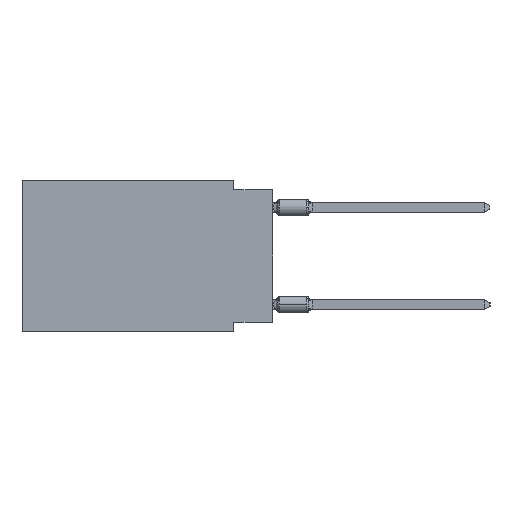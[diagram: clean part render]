
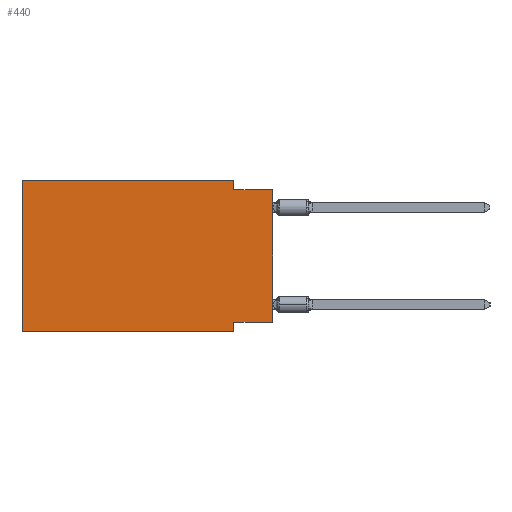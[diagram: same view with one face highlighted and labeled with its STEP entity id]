
A CAD part, left-side view. The second image highlights one B-rep face of the part: STEP entity #440.
In plain terms, the highlighted planar face has unit normal (-1, 0, 0).
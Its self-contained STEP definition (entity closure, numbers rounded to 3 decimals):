
#440 = ADVANCED_FACE ( 'NONE', ( #2501 ), #32997, .F. ) ;
#1200 = LINE ( 'NONE', #47412, #42851 ) ;
#1659 = DIRECTION ( 'NONE',  ( 0., 0., 1. ) ) ;
#2501 = FACE_OUTER_BOUND ( 'NONE', #46681, .T. ) ;
#2604 = CARTESIAN_POINT ( 'NONE',  ( 0., 16.383, 0. ) ) ;
#3352 = VERTEX_POINT ( 'NONE', #38070 ) ;
#3527 = CARTESIAN_POINT ( 'NONE',  ( 0., 0., -9.271 ) ) ;
#3734 = VECTOR ( 'NONE', #30054, 1000. ) ;
#4152 = DIRECTION ( 'NONE',  ( 0., -1., 0. ) ) ;
#4276 = EDGE_CURVE ( 'NONE', #45955, #41901, #1200, .T. ) ;
#6982 = VECTOR ( 'NONE', #19776, 1000. ) ;
#7915 = LINE ( 'NONE', #23152, #16522 ) ;
#9333 = ORIENTED_EDGE ( 'NONE', *, *, #24604, .F. ) ;
#11074 = EDGE_CURVE ( 'NONE', #18212, #33989, #23517, .T. ) ;
#11543 = LINE ( 'NONE', #37766, #3734 ) ;
#12937 = LINE ( 'NONE', #35908, #48739 ) ;
#13094 = EDGE_CURVE ( 'NONE', #32169, #45270, #7915, .T. ) ;
#13452 = LINE ( 'NONE', #28693, #17231 ) ;
#13585 = VECTOR ( 'NONE', #48039, 1000. ) ;
#15431 = EDGE_CURVE ( 'NONE', #18212, #45270, #12937, .T. ) ;
#15571 = CARTESIAN_POINT ( 'NONE',  ( 0., 2.54, 0. ) ) ;
#16522 = VECTOR ( 'NONE', #4152, 1000. ) ;
#16866 = ORIENTED_EDGE ( 'NONE', *, *, #45323, .T. ) ;
#17231 = VECTOR ( 'NONE', #43908, 1000. ) ;
#17583 = LINE ( 'NONE', #32808, #13585 ) ;
#18212 = VERTEX_POINT ( 'NONE', #36369 ) ;
#19776 = DIRECTION ( 'NONE',  ( 0., 1., 0. ) ) ;
#21124 = ORIENTED_EDGE ( 'NONE', *, *, #15431, .T. ) ;
#21725 = CARTESIAN_POINT ( 'NONE',  ( 0., 16.383, 0. ) ) ;
#21810 = VECTOR ( 'NONE', #22114, 1000. ) ;
#21903 = VERTEX_POINT ( 'NONE', #35056 ) ;
#22114 = DIRECTION ( 'NONE',  ( 0., 0., 1. ) ) ;
#23152 = CARTESIAN_POINT ( 'NONE',  ( 0., 0., -0.635 ) ) ;
#23450 = EDGE_CURVE ( 'NONE', #33989, #3352, #11543, .T. ) ;
#23517 = LINE ( 'NONE', #3527, #6982 ) ;
#23766 = CARTESIAN_POINT ( 'NONE',  ( 0., 0., -0.635 ) ) ;
#24604 = EDGE_CURVE ( 'NONE', #41901, #32169, #17583, .T. ) ;
#25122 = LINE ( 'NONE', #2604, #21810 ) ;
#27150 = CARTESIAN_POINT ( 'NONE',  ( 0., 2.54, -0.635 ) ) ;
#27829 = ORIENTED_EDGE ( 'NONE', *, *, #11074, .F. ) ;
#28693 = CARTESIAN_POINT ( 'NONE',  ( 0., 16.383, -9.906 ) ) ;
#30054 = DIRECTION ( 'NONE',  ( 0., 0., -1. ) ) ;
#31110 = ORIENTED_EDGE ( 'NONE', *, *, #36516, .F. ) ;
#32169 = VERTEX_POINT ( 'NONE', #27150 ) ;
#32808 = CARTESIAN_POINT ( 'NONE',  ( 0., 2.54, 0. ) ) ;
#32997 = PLANE ( 'NONE',  #45422 ) ;
#33724 = DIRECTION ( 'NONE',  ( 0., 0., -1. ) ) ;
#33989 = VERTEX_POINT ( 'NONE', #48510 ) ;
#35056 = CARTESIAN_POINT ( 'NONE',  ( 0., 16.383, -9.906 ) ) ;
#35908 = CARTESIAN_POINT ( 'NONE',  ( 0., 0., 0. ) ) ;
#36369 = CARTESIAN_POINT ( 'NONE',  ( 0., 0., -9.271 ) ) ;
#36516 = EDGE_CURVE ( 'NONE', #21903, #45955, #25122, .T. ) ;
#37475 = CARTESIAN_POINT ( 'NONE',  ( 0., 16.383, 0. ) ) ;
#37766 = CARTESIAN_POINT ( 'NONE',  ( 0., 2.54, -9.906 ) ) ;
#38070 = CARTESIAN_POINT ( 'NONE',  ( 0., 2.54, -9.906 ) ) ;
#38974 = ORIENTED_EDGE ( 'NONE', *, *, #13094, .F. ) ;
#39178 = DIRECTION ( 'NONE',  ( 0., -1., 0. ) ) ;
#41458 = DIRECTION ( 'NONE',  ( 1., 0., 0. ) ) ;
#41901 = VERTEX_POINT ( 'NONE', #15571 ) ;
#42851 = VECTOR ( 'NONE', #39178, 1000. ) ;
#43004 = ORIENTED_EDGE ( 'NONE', *, *, #4276, .F. ) ;
#43908 = DIRECTION ( 'NONE',  ( 0., -1., 0. ) ) ;
#45270 = VERTEX_POINT ( 'NONE', #23766 ) ;
#45323 = EDGE_CURVE ( 'NONE', #21903, #3352, #13452, .T. ) ;
#45422 = AXIS2_PLACEMENT_3D ( 'NONE', #37475, #41458, #33724 ) ;
#45955 = VERTEX_POINT ( 'NONE', #21725 ) ;
#46117 = ORIENTED_EDGE ( 'NONE', *, *, #23450, .F. ) ;
#46681 = EDGE_LOOP ( 'NONE', ( #21124, #38974, #9333, #43004, #31110, #16866, #46117, #27829 ) ) ;
#47412 = CARTESIAN_POINT ( 'NONE',  ( 0., 16.383, 0. ) ) ;
#48039 = DIRECTION ( 'NONE',  ( 0., 0., -1. ) ) ;
#48510 = CARTESIAN_POINT ( 'NONE',  ( 0., 2.54, -9.271 ) ) ;
#48739 = VECTOR ( 'NONE', #1659, 1000. ) ;
